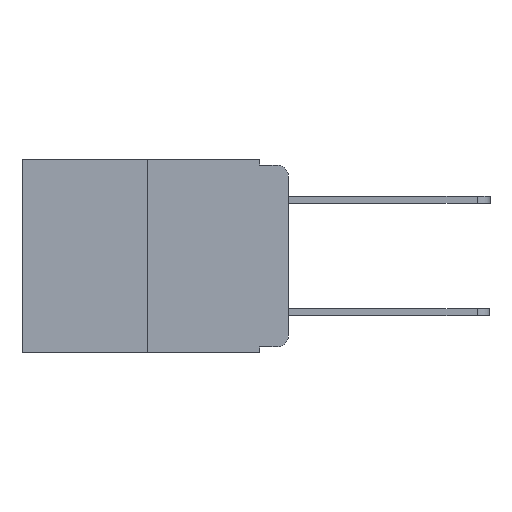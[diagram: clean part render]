
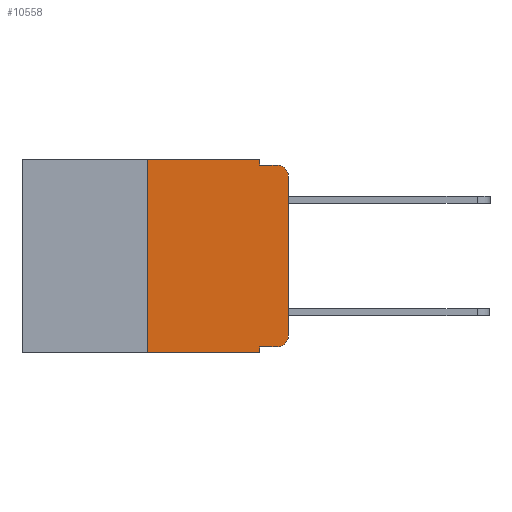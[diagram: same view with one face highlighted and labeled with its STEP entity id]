
A CAD part, left-side view. The second image highlights one B-rep face of the part: STEP entity #10558.
In plain terms, the highlighted planar face has unit normal (-1, 0, 0).
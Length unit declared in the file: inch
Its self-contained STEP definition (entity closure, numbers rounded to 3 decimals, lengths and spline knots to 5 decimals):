
#94 = DIRECTION ( 'NONE',  ( 0., 0., -1. ) ) ;
#349 = DIRECTION ( 'NONE',  ( 0., 0., 1. ) ) ;
#449 = CARTESIAN_POINT ( 'NONE',  ( 0., 0.25, 0. ) ) ;
#1073 = EDGE_LOOP ( 'NONE', ( #4803, #11346, #7789, #13224, #9679, #3664, #5569, #2643, #9675, #12970 ) ) ;
#1349 = CARTESIAN_POINT ( 'NONE',  ( 0., 0.02, -0.01 ) ) ;
#2002 = CARTESIAN_POINT ( 'NONE',  ( 0., 0., 0. ) ) ;
#2484 = EDGE_CURVE ( 'NONE', #21556, #10924, #7829, .T. ) ;
#2643 = ORIENTED_EDGE ( 'NONE', *, *, #19917, .F. ) ;
#3664 = ORIENTED_EDGE ( 'NONE', *, *, #9619, .F. ) ;
#3883 = CARTESIAN_POINT ( 'NONE',  ( 0., 0.051, -0.01 ) ) ;
#4115 = VECTOR ( 'NONE', #12856, 39.37008 ) ;
#4127 = CARTESIAN_POINT ( 'NONE',  ( 0., 0.051, 0. ) ) ;
#4803 = ORIENTED_EDGE ( 'NONE', *, *, #15050, .T. ) ;
#5187 = LINE ( 'NONE', #11090, #4115 ) ;
#5427 = CARTESIAN_POINT ( 'NONE',  ( 0., 0.051, -0.333 ) ) ;
#5503 = DIRECTION ( 'NONE',  ( 0., -1., 0. ) ) ;
#5569 = ORIENTED_EDGE ( 'NONE', *, *, #2484, .T. ) ;
#5616 = DIRECTION ( 'NONE',  ( 0., -1., 0. ) ) ;
#5872 = DIRECTION ( 'NONE',  ( 0., 0., -1. ) ) ;
#6258 = VERTEX_POINT ( 'NONE', #17792 ) ;
#6390 = VECTOR ( 'NONE', #7892, 39.37008 ) ;
#6471 = VERTEX_POINT ( 'NONE', #11637 ) ;
#6516 = VERTEX_POINT ( 'NONE', #1349 ) ;
#6524 = DIRECTION ( 'NONE',  ( 1., 0., 0. ) ) ;
#6610 = VERTEX_POINT ( 'NONE', #15317 ) ;
#6877 = DIRECTION ( 'NONE',  ( -1., 0., 0. ) ) ;
#7079 = VERTEX_POINT ( 'NONE', #18493 ) ;
#7245 = VECTOR ( 'NONE', #16711, 39.37008 ) ;
#7354 = CARTESIAN_POINT ( 'NONE',  ( 0., 0.473, -0.343 ) ) ;
#7637 = VECTOR ( 'NONE', #5503, 39.37008 ) ;
#7789 = ORIENTED_EDGE ( 'NONE', *, *, #21978, .F. ) ;
#7829 = LINE ( 'NONE', #7354, #16346 ) ;
#7892 = DIRECTION ( 'NONE',  ( 0., 0., 1. ) ) ;
#7970 = LINE ( 'NONE', #4127, #13076 ) ;
#8433 = EDGE_CURVE ( 'NONE', #13326, #6258, #16327, .T. ) ;
#8731 = VERTEX_POINT ( 'NONE', #449 ) ;
#9255 = CARTESIAN_POINT ( 'NONE',  ( 0., 0.051, -0.343 ) ) ;
#9619 = EDGE_CURVE ( 'NONE', #21556, #8731, #11009, .T. ) ;
#9664 = CARTESIAN_POINT ( 'NONE',  ( 0., 0.25, 0. ) ) ;
#9675 = ORIENTED_EDGE ( 'NONE', *, *, #12640, .T. ) ;
#9679 = ORIENTED_EDGE ( 'NONE', *, *, #12203, .F. ) ;
#10210 = DIRECTION ( 'NONE',  ( 0., -1., 0. ) ) ;
#10457 = DIRECTION ( 'NONE',  ( -1., 0., 0. ) ) ;
#10558 = ADVANCED_FACE ( 'NONE', ( #11507 ), #13366, .F. ) ;
#10689 = CIRCLE ( 'NONE', #13494, 0.02 ) ;
#10881 = VECTOR ( 'NONE', #349, 39.37008 ) ;
#10924 = VERTEX_POINT ( 'NONE', #9255 ) ;
#11009 = LINE ( 'NONE', #9664, #6390 ) ;
#11090 = CARTESIAN_POINT ( 'NONE',  ( 0., 0.473, 0. ) ) ;
#11346 = ORIENTED_EDGE ( 'NONE', *, *, #19789, .T. ) ;
#11507 = FACE_OUTER_BOUND ( 'NONE', #1073, .T. ) ;
#11637 = CARTESIAN_POINT ( 'NONE',  ( 0., 0.02, -0.333 ) ) ;
#11726 = VERTEX_POINT ( 'NONE', #16179 ) ;
#12203 = EDGE_CURVE ( 'NONE', #8731, #13326, #5187, .T. ) ;
#12640 = EDGE_CURVE ( 'NONE', #6610, #6471, #21118, .T. ) ;
#12735 = VECTOR ( 'NONE', #5616, 39.37008 ) ;
#12856 = DIRECTION ( 'NONE',  ( 0., -1., 0. ) ) ;
#12970 = ORIENTED_EDGE ( 'NONE', *, *, #21788, .T. ) ;
#13076 = VECTOR ( 'NONE', #5872, 39.37008 ) ;
#13224 = ORIENTED_EDGE ( 'NONE', *, *, #8433, .F. ) ;
#13270 = LINE ( 'NONE', #3883, #12735 ) ;
#13326 = VERTEX_POINT ( 'NONE', #15800 ) ;
#13366 = PLANE ( 'NONE',  #21731 ) ;
#13494 = AXIS2_PLACEMENT_3D ( 'NONE', #20487, #10457, #94 ) ;
#14374 = AXIS2_PLACEMENT_3D ( 'NONE', #17051, #6877, #18733 ) ;
#15050 = EDGE_CURVE ( 'NONE', #7079, #11726, #15376, .T. ) ;
#15317 = CARTESIAN_POINT ( 'NONE',  ( 0., 0.051, -0.333 ) ) ;
#15376 = LINE ( 'NONE', #2002, #10881 ) ;
#15800 = CARTESIAN_POINT ( 'NONE',  ( 0., 0.051, 0. ) ) ;
#16179 = CARTESIAN_POINT ( 'NONE',  ( 0., 0., -0.03 ) ) ;
#16327 = LINE ( 'NONE', #21723, #7245 ) ;
#16346 = VECTOR ( 'NONE', #10210, 39.37008 ) ;
#16711 = DIRECTION ( 'NONE',  ( 0., 0., -1. ) ) ;
#16733 = CARTESIAN_POINT ( 'NONE',  ( 0., 0.473, 0. ) ) ;
#17051 = CARTESIAN_POINT ( 'NONE',  ( 0., 0.02, -0.313 ) ) ;
#17792 = CARTESIAN_POINT ( 'NONE',  ( 0., 0.051, -0.01 ) ) ;
#18419 = DIRECTION ( 'NONE',  ( 0., 0., -1. ) ) ;
#18493 = CARTESIAN_POINT ( 'NONE',  ( 0., 0., -0.313 ) ) ;
#18733 = DIRECTION ( 'NONE',  ( 0., 0., -1. ) ) ;
#19771 = CARTESIAN_POINT ( 'NONE',  ( 0., 0.25, -0.343 ) ) ;
#19789 = EDGE_CURVE ( 'NONE', #11726, #6516, #10689, .T. ) ;
#19917 = EDGE_CURVE ( 'NONE', #6610, #10924, #7970, .T. ) ;
#20487 = CARTESIAN_POINT ( 'NONE',  ( 0., 0.02, -0.03 ) ) ;
#21118 = LINE ( 'NONE', #5427, #7637 ) ;
#21372 = CIRCLE ( 'NONE', #14374, 0.02 ) ;
#21556 = VERTEX_POINT ( 'NONE', #19771 ) ;
#21723 = CARTESIAN_POINT ( 'NONE',  ( 0., 0.051, 0. ) ) ;
#21731 = AXIS2_PLACEMENT_3D ( 'NONE', #16733, #6524, #18419 ) ;
#21788 = EDGE_CURVE ( 'NONE', #6471, #7079, #21372, .T. ) ;
#21978 = EDGE_CURVE ( 'NONE', #6258, #6516, #13270, .T. ) ;
